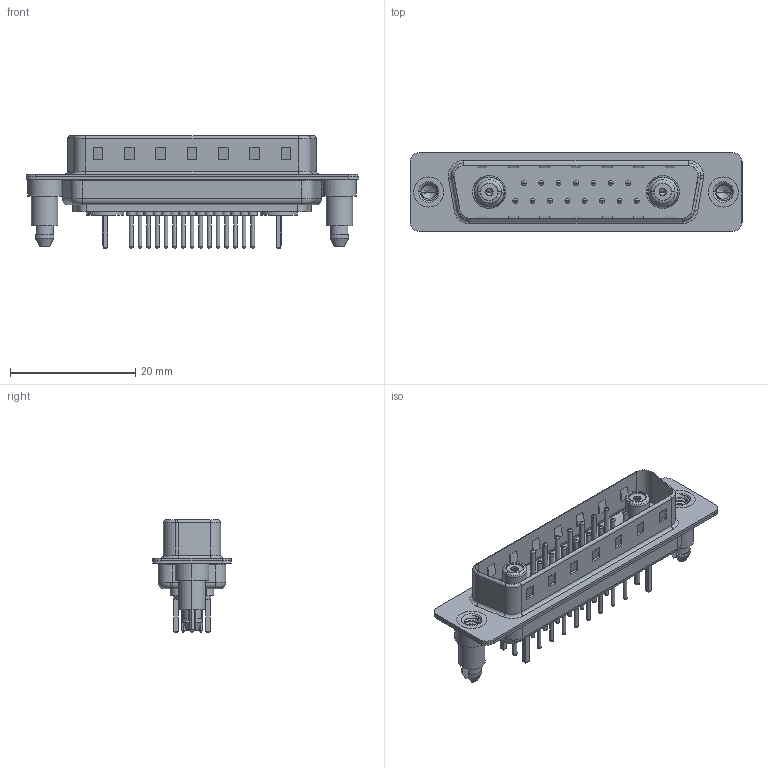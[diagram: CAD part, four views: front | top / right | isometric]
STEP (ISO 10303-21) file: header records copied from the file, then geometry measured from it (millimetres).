
FILE_DESCRIPTION (( 'STEP AP203' ), '1' );
FILE_NAME ('627-17W2224-5T5.STEP', '2019-05-27T21:33:03', ( '' ), ( '' ), 'SwSTEP 2.0', 'SolidWorks 2016', '' );
FILE_SCHEMA (( 'CONFIG_CONTROL_DESIGN' ));
Length unit declared in the file: millimetre
Products named in the file (13): Co-Ax Jack_Straight PC Tail; Insulator Socket 2; 627Combo Housing_17W2; 627Combo Shell Front_25 Contacts; Insulator Socket; 627Combo Contact Row 1_24; Locking Collar; Co-Ax Jack Assy_S; 627Combo Threaded Boardlock_5; Socket_Str; 627Combo Contact Row 2_24; 627-17W2224-5T5; 627Combo Shell Rear_25 Contacts
Assembly tree (27 placements, depth 3):
  627-17W2224-5T5
    627Combo Housing_17W2
    627Combo Shell Rear_25 Contacts
    627Combo Shell Front_25 Contacts
    627Combo Threaded Boardlock_5  x2
    Co-Ax Jack Assy_S  x2
      Co-Ax Jack_Straight PC Tail
      Insulator Socket
      Insulator Socket 2
      Locking Collar
      Socket_Str
    627Combo Contact Row 1_24  x7
    627Combo Contact Row 2_24  x8
Bounding box: 53 x 12.6 x 17.9 mm (x, y, z)
Volume: 2895.6 mm3; surface area: 7930.6 mm2
Topology: 30 solids, 30 shells, 1203 faces, 2697 edges, 1660 vertices
Faces by surface type: cylinder 473, plane 386, torus 298, cone 32, bspline 10, sphere 4
Entity records: 22900 total; most frequent: CARTESIAN_POINT 5129, DIRECTION 3572, ORIENTED_EDGE 3154, EDGE_CURVE 1577, AXIS2_PLACEMENT_3D 1391, VERTEX_POINT 1001, EDGE_LOOP 806, VECTOR 790
